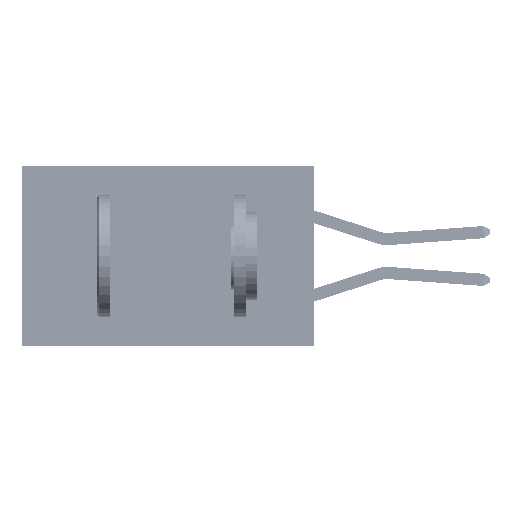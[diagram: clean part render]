
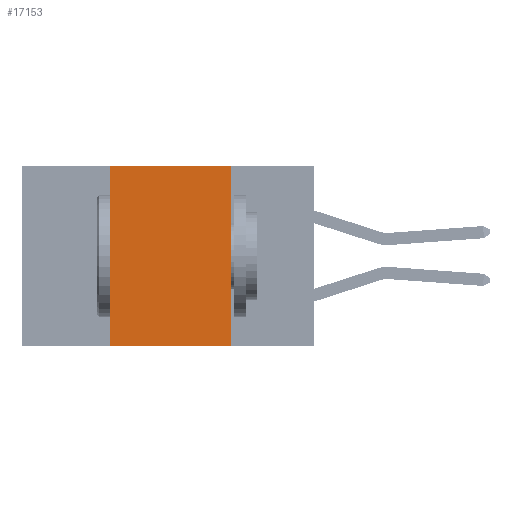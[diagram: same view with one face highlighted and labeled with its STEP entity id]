
A CAD part, left-side view. The second image highlights one B-rep face of the part: STEP entity #17153.
In plain terms, the highlighted planar face has unit normal (-1, 0, 0).
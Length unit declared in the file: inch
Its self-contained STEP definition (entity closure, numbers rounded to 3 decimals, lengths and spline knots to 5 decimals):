
#1633 = VERTEX_POINT ( 'NONE', #20007 ) ;
#1671 = VECTOR ( 'NONE', #24266, 39.37008 ) ;
#2281 = ORIENTED_EDGE ( 'NONE', *, *, #19001, .F. ) ;
#3885 = EDGE_CURVE ( 'NONE', #13506, #1633, #37977, .T. ) ;
#4563 = ORIENTED_EDGE ( 'NONE', *, *, #12757, .T. ) ;
#9021 = PLANE ( 'NONE',  #20593 ) ;
#10514 = CARTESIAN_POINT ( 'NONE',  ( 0., 0.17, 0. ) ) ;
#12654 = DIRECTION ( 'NONE',  ( 1., 0., 0. ) ) ;
#12757 = EDGE_CURVE ( 'NONE', #41216, #1633, #20842, .T. ) ;
#12902 = VERTEX_POINT ( 'NONE', #46135 ) ;
#13506 = VERTEX_POINT ( 'NONE', #24516 ) ;
#14140 = DIRECTION ( 'NONE',  ( 0., 0., -1. ) ) ;
#17043 = CARTESIAN_POINT ( 'NONE',  ( 0., 0.6, -0.37 ) ) ;
#17153 = ADVANCED_FACE ( 'NONE', ( #20565 ), #9021, .F. ) ;
#19001 = EDGE_CURVE ( 'NONE', #41216, #12902, #35818, .T. ) ;
#19963 = VECTOR ( 'NONE', #39099, 39.37008 ) ;
#20007 = CARTESIAN_POINT ( 'NONE',  ( 0., 0.17, -0.37 ) ) ;
#20213 = VECTOR ( 'NONE', #14140, 39.37008 ) ;
#20565 = FACE_OUTER_BOUND ( 'NONE', #38273, .T. ) ;
#20593 = AXIS2_PLACEMENT_3D ( 'NONE', #34067, #12654, #37583 ) ;
#20842 = LINE ( 'NONE', #17043, #1671 ) ;
#24266 = DIRECTION ( 'NONE',  ( 0., -1., 0. ) ) ;
#24516 = CARTESIAN_POINT ( 'NONE',  ( 0., 0.17, 0. ) ) ;
#25917 = EDGE_CURVE ( 'NONE', #12902, #13506, #29521, .T. ) ;
#29521 = LINE ( 'NONE', #46134, #19963 ) ;
#31730 = DIRECTION ( 'NONE',  ( 0., 0., 1. ) ) ;
#34067 = CARTESIAN_POINT ( 'NONE',  ( 0., 0.6, 0. ) ) ;
#34806 = ORIENTED_EDGE ( 'NONE', *, *, #3885, .F. ) ;
#35818 = LINE ( 'NONE', #42160, #44014 ) ;
#35917 = ORIENTED_EDGE ( 'NONE', *, *, #25917, .F. ) ;
#37583 = DIRECTION ( 'NONE',  ( 0., 0., -1. ) ) ;
#37977 = LINE ( 'NONE', #10514, #20213 ) ;
#38273 = EDGE_LOOP ( 'NONE', ( #34806, #35917, #2281, #4563 ) ) ;
#39099 = DIRECTION ( 'NONE',  ( 0., -1., 0. ) ) ;
#39548 = CARTESIAN_POINT ( 'NONE',  ( 0., 0.42, -0.37 ) ) ;
#41216 = VERTEX_POINT ( 'NONE', #39548 ) ;
#42160 = CARTESIAN_POINT ( 'NONE',  ( 0., 0.42, 0. ) ) ;
#44014 = VECTOR ( 'NONE', #31730, 39.37008 ) ;
#46134 = CARTESIAN_POINT ( 'NONE',  ( 0., 0.6, 0. ) ) ;
#46135 = CARTESIAN_POINT ( 'NONE',  ( 0., 0.42, 0. ) ) ;
